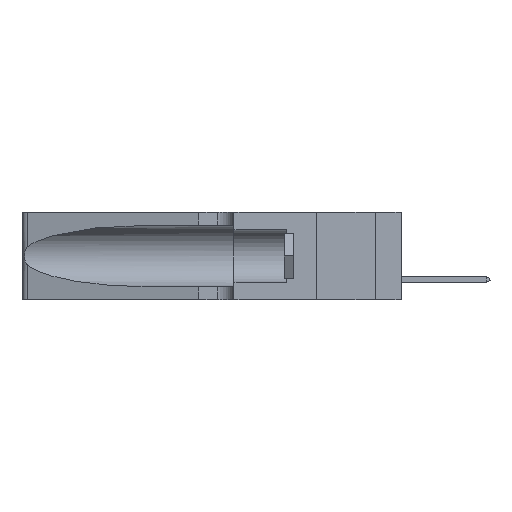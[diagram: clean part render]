
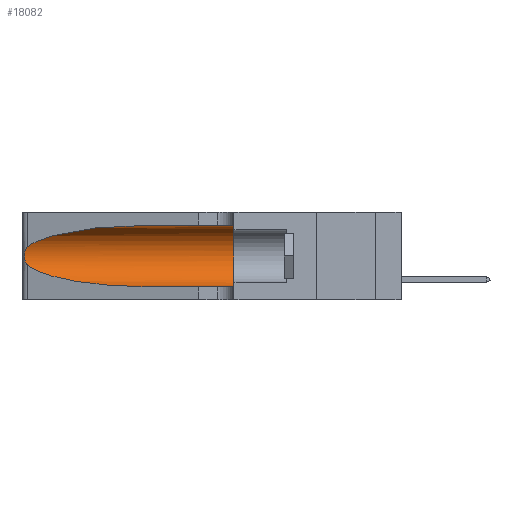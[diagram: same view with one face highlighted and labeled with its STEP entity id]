
A CAD part, left-side view. The second image highlights one B-rep face of the part: STEP entity #18082.
In plain terms, the highlighted cylindrical face has radius 3.308 mm (diameter 6.617 mm), a partial arc.
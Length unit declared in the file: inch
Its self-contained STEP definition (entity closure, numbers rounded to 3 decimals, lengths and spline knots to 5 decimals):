
#199 = CARTESIAN_POINT ( 'NONE',  ( 0.1305, 0.35, 0.31525 ) ) ;
#520 = DIRECTION ( 'NONE',  ( 0., -1., 0. ) ) ;
#685 = EDGE_CURVE ( 'NONE', #8822, #3898, #17893, .T. ) ;
#1040 = EDGE_LOOP ( 'NONE', ( #15787, #9033, #18541, #18412, #1657, #17799 ) ) ;
#1060 = AXIS2_PLACEMENT_3D ( 'NONE', #13890, #6277, #16923 ) ;
#1657 = ORIENTED_EDGE ( 'NONE', *, *, #2335, .F. ) ;
#1814 = VERTEX_POINT ( 'NONE', #12457 ) ;
#2069 = CARTESIAN_POINT ( 'NONE',  ( 0.1305, 0.35, 0.185 ) ) ;
#2212 = VERTEX_POINT ( 'NONE', #199 ) ;
#2335 = EDGE_CURVE ( 'NONE', #2212, #1814, #10717, .T. ) ;
#2974 = CARTESIAN_POINT ( 'NONE',  ( 0.25555, 1.22993, 0.14849 ) ) ;
#3041 = CARTESIAN_POINT ( 'NONE',  ( 0.25487, 1.22718, 0.14631 ) ) ;
#3164 = CARTESIAN_POINT ( 'NONE',  ( 0.25487, 1.22718, 0.22369 ) ) ;
#3305 = CARTESIAN_POINT ( 'NONE',  ( 0.1305, 0.72297, 0.05475 ) ) ;
#3898 = VERTEX_POINT ( 'NONE', #9616 ) ;
#4114 = CARTESIAN_POINT ( 'NONE',  ( 0.25787, 1.23484, 0.2124 ) ) ;
#4219 = CYLINDRICAL_SURFACE ( 'NONE', #1060, 0.13025 ) ;
#4430 = AXIS2_PLACEMENT_3D ( 'NONE', #2069, #8422, #11474 ) ;
#4446 = CARTESIAN_POINT ( 'NONE',  ( 0.1305, 0.72297, 0.31525 ) ) ;
#4978 = CARTESIAN_POINT ( 'NONE',  ( 0.25487, 1.22718, 0.14631 ) ) ;
#5632 = CARTESIAN_POINT ( 'NONE',  ( 0.25639, 1.23186, 0.15144 ) ) ;
#5781 = EDGE_CURVE ( 'NONE', #8112, #1814, #9031, .T. ) ;
#6040 = CARTESIAN_POINT ( 'NONE',  ( 0.2373, 1.15595, 0.28018 ) ) ;
#6063 = B_SPLINE_CURVE_WITH_KNOTS ( 'NONE', 3,
 ( #3164, #19345, #16741, #4114, #9106, #7634, #10248, #14776, #16279, #12109, #18226, #5632, #2974, #3041 ),
 .UNSPECIFIED., .F., .F.,
 ( 4, 2, 2, 2, 2, 2, 4 ),
 ( 0., 0.00027, 0.00053, 0.00107, 0.0016, 0.00187, 0.00214 ),
 .UNSPECIFIED. ) ;
#6277 = DIRECTION ( 'NONE',  ( 0., -1., 0. ) ) ;
#6626 = VECTOR ( 'NONE', #520, 39.37008 ) ;
#7634 = CARTESIAN_POINT ( 'NONE',  ( 0.26018, 1.23835, 0.19895 ) ) ;
#8112 = VERTEX_POINT ( 'NONE', #9516 ) ;
#8422 = DIRECTION ( 'NONE',  ( 0., 1., 0. ) ) ;
#8822 = VERTEX_POINT ( 'NONE', #11970 ) ;
#9031 = LINE ( 'NONE', #18764, #6626 ) ;
#9033 = ORIENTED_EDGE ( 'NONE', *, *, #14843, .T. ) ;
#9106 = CARTESIAN_POINT ( 'NONE',  ( 0.25854, 1.2359, 0.20912 ) ) ;
#9237 = VECTOR ( 'NONE', #13004, 39.37008 ) ;
#9247 = CARTESIAN_POINT ( 'NONE',  ( 0.18966, 0.96281, 0.05475 ) ) ;
#9516 = CARTESIAN_POINT ( 'NONE',  ( 0.1305, 0.72297, 0.05475 ) ) ;
#9616 = CARTESIAN_POINT ( 'NONE',  ( 0.25487, 1.22718, 0.22369 ) ) ;
#10248 = CARTESIAN_POINT ( 'NONE',  ( 0.26075, 1.23896, 0.19203 ) ) ;
#10649 = CARTESIAN_POINT ( 'NONE',  ( 0.25487, 1.22718, 0.22369 ) ) ;
#10717 = CIRCLE ( 'NONE', #4430, 0.13025 ) ;
#10774 = CARTESIAN_POINT ( 'NONE',  ( 0.18966, 0.96281, 0.31525 ) ) ;
#11161 = LINE ( 'NONE', #13071, #9237 ) ;
#11474 = DIRECTION ( 'NONE',  ( 0., 0., 1. ) ) ;
#11970 = CARTESIAN_POINT ( 'NONE',  ( 0.1305, 0.72297, 0.31525 ) ) ;
#12109 = CARTESIAN_POINT ( 'NONE',  ( 0.25856, 1.23593, 0.16098 ) ) ;
#12457 = CARTESIAN_POINT ( 'NONE',  ( 0.1305, 0.35, 0.05475 ) ) ;
#12523 = CARTESIAN_POINT ( 'NONE',  ( 0.2373, 1.15595, 0.08982 ) ) ;
#13004 = DIRECTION ( 'NONE',  ( 0., -1., 0. ) ) ;
#13071 = CARTESIAN_POINT ( 'NONE',  ( 0.1305, 1.61858, 0.31525 ) ) ;
#13448 = EDGE_CURVE ( 'NONE', #8822, #2212, #11161, .T. ) ;
#13890 = CARTESIAN_POINT ( 'NONE',  ( 0.1305, 1.61858, 0.185 ) ) ;
#14776 = CARTESIAN_POINT ( 'NONE',  ( 0.26075, 1.23896, 0.178 ) ) ;
#14843 = EDGE_CURVE ( 'NONE', #3898, #16822, #6063, .T. ) ;
#15787 = ORIENTED_EDGE ( 'NONE', *, *, #685, .T. ) ;
#16279 = CARTESIAN_POINT ( 'NONE',  ( 0.26017, 1.23833, 0.17102 ) ) ;
#16350 = FACE_OUTER_BOUND ( 'NONE', #1040, .T. ) ;
#16741 = CARTESIAN_POINT ( 'NONE',  ( 0.25639, 1.23184, 0.21858 ) ) ;
#16822 = VERTEX_POINT ( 'NONE', #18695 ) ;
#16923 = DIRECTION ( 'NONE',  ( 0., 0., -1. ) ) ;
#17271 =( BOUNDED_CURVE ( )  B_SPLINE_CURVE ( 3, ( #4978, #12523, #9247, #3305 ),
 .UNSPECIFIED., .F., .T. ) 
 B_SPLINE_CURVE_WITH_KNOTS ( ( 4, 4 ),
 ( 3.44316, 4.71239 ),
 .UNSPECIFIED. ) 
 CURVE ( )  GEOMETRIC_REPRESENTATION_ITEM ( )  RATIONAL_B_SPLINE_CURVE ( ( 1., 0.87, 0.87, 1. ) ) 
 REPRESENTATION_ITEM ( '' )  );
#17799 = ORIENTED_EDGE ( 'NONE', *, *, #13448, .F. ) ;
#17893 =( BOUNDED_CURVE ( )  B_SPLINE_CURVE ( 3, ( #4446, #10774, #6040, #10649 ),
 .UNSPECIFIED., .F., .F. ) 
 B_SPLINE_CURVE_WITH_KNOTS ( ( 4, 4 ),
 ( 1.5708, 2.84003 ),
 .UNSPECIFIED. ) 
 CURVE ( )  GEOMETRIC_REPRESENTATION_ITEM ( )  RATIONAL_B_SPLINE_CURVE ( ( 1., 0.87, 0.87, 1. ) ) 
 REPRESENTATION_ITEM ( '' )  );
#18082 = ADVANCED_FACE ( 'NONE', ( #16350 ), #4219, .F. ) ;
#18226 = CARTESIAN_POINT ( 'NONE',  ( 0.25789, 1.23486, 0.15765 ) ) ;
#18412 = ORIENTED_EDGE ( 'NONE', *, *, #5781, .T. ) ;
#18541 = ORIENTED_EDGE ( 'NONE', *, *, #19398, .T. ) ;
#18695 = CARTESIAN_POINT ( 'NONE',  ( 0.25487, 1.22718, 0.14631 ) ) ;
#18764 = CARTESIAN_POINT ( 'NONE',  ( 0.1305, 1.61858, 0.05475 ) ) ;
#19345 = CARTESIAN_POINT ( 'NONE',  ( 0.25555, 1.22994, 0.2215 ) ) ;
#19398 = EDGE_CURVE ( 'NONE', #16822, #8112, #17271, .T. ) ;
